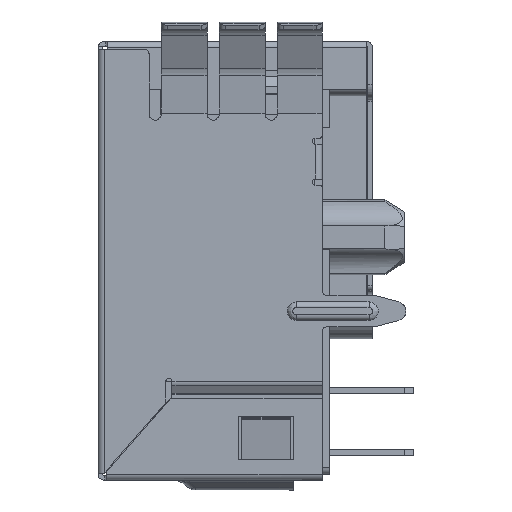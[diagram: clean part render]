
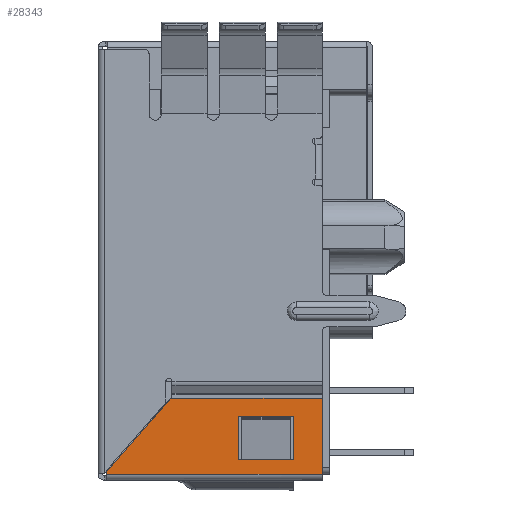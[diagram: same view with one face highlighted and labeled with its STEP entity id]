
A CAD part, left-side view. The second image highlights one B-rep face of the part: STEP entity #28343.
In plain terms, the highlighted planar face has unit normal (-1, 0, 0).
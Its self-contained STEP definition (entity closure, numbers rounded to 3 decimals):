
#635 = DIRECTION ( 'NONE',  ( 0., 0., -1. ) ) ;
#723 = DIRECTION ( 'NONE',  ( 0., 0., 1. ) ) ;
#1382 = CARTESIAN_POINT ( 'NONE',  ( -7.52, 2.664, -5.675 ) ) ;
#1685 = DIRECTION ( 'NONE',  ( 0., 1., 0. ) ) ;
#2190 = DIRECTION ( 'NONE',  ( 0., -1., 0. ) ) ;
#2287 = DIRECTION ( 'NONE',  ( 0., -0.656, 0.755 ) ) ;
#2472 = ORIENTED_EDGE ( 'NONE', *, *, #31273, .F. ) ;
#3243 = FACE_BOUND ( 'NONE', #34514, .T. ) ;
#3297 = CARTESIAN_POINT ( 'NONE',  ( -7.52, -3.595, -7.25 ) ) ;
#3355 = VERTEX_POINT ( 'NONE', #1382 ) ;
#3438 = ORIENTED_EDGE ( 'NONE', *, *, #42101, .F. ) ;
#4588 = EDGE_CURVE ( 'NONE', #16479, #9830, #34525, .T. ) ;
#4747 = ORIENTED_EDGE ( 'NONE', *, *, #38021, .F. ) ;
#5035 = VECTOR ( 'NONE', #635, 1000. ) ;
#5371 = CARTESIAN_POINT ( 'NONE',  ( -7.52, 0.86, -8.225 ) ) ;
#5658 = LINE ( 'NONE', #30235, #27336 ) ;
#8617 = LINE ( 'NONE', #3297, #37883 ) ;
#9566 = CARTESIAN_POINT ( 'NONE',  ( -7.52, 5.382, -8.802 ) ) ;
#9830 = VERTEX_POINT ( 'NONE', #13491 ) ;
#10467 = ORIENTED_EDGE ( 'NONE', *, *, #23598, .F. ) ;
#12222 = VERTEX_POINT ( 'NONE', #24461 ) ;
#12739 = VERTEX_POINT ( 'NONE', #41250 ) ;
#13322 = CARTESIAN_POINT ( 'NONE',  ( -7.52, 5.315, -8.725 ) ) ;
#13491 = CARTESIAN_POINT ( 'NONE',  ( -7.52, -3.595, -8.825 ) ) ;
#14231 = CARTESIAN_POINT ( 'NONE',  ( -7.52, -2.425, -7.25 ) ) ;
#14497 = CARTESIAN_POINT ( 'NONE',  ( -7.52, 5.315, -7.25 ) ) ;
#15833 = CARTESIAN_POINT ( 'NONE',  ( -7.52, -0.125, -6.425 ) ) ;
#16479 = VERTEX_POINT ( 'NONE', #30899 ) ;
#18339 = CARTESIAN_POINT ( 'NONE',  ( -7.52, 0.91, -8.825 ) ) ;
#19613 = VERTEX_POINT ( 'NONE', #21923 ) ;
#19682 = VERTEX_POINT ( 'NONE', #15833 ) ;
#20424 = CARTESIAN_POINT ( 'NONE',  ( -7.52, 0.86, -6.425 ) ) ;
#20758 = LINE ( 'NONE', #28058, #5035 ) ;
#21678 = LINE ( 'NONE', #9566, #28191 ) ;
#21785 = ORIENTED_EDGE ( 'NONE', *, *, #25831, .F. ) ;
#21923 = CARTESIAN_POINT ( 'NONE',  ( -7.52, -2.425, -8.225 ) ) ;
#23598 = EDGE_CURVE ( 'NONE', #12739, #19682, #28044, .T. ) ;
#24461 = CARTESIAN_POINT ( 'NONE',  ( -7.52, -3.595, -5.675 ) ) ;
#25352 = AXIS2_PLACEMENT_3D ( 'NONE', #26102, #36106, #1685 ) ;
#25679 = DIRECTION ( 'NONE',  ( 0., -1., 0. ) ) ;
#25831 = EDGE_CURVE ( 'NONE', #19613, #12739, #38801, .T. ) ;
#26102 = CARTESIAN_POINT ( 'NONE',  ( -7.52, -3.773, -8.888 ) ) ;
#26449 = VECTOR ( 'NONE', #723, 1000. ) ;
#26866 = EDGE_CURVE ( 'NONE', #19682, #30951, #20758, .T. ) ;
#27336 = VECTOR ( 'NONE', #2190, 1000. ) ;
#28044 = LINE ( 'NONE', #20424, #38394 ) ;
#28058 = CARTESIAN_POINT ( 'NONE',  ( -7.52, -0.125, -7.25 ) ) ;
#28191 = VECTOR ( 'NONE', #2287, 1000. ) ;
#28343 = ADVANCED_FACE ( 'NONE', ( #3243, #42855 ), #39617, .F. ) ;
#28553 = EDGE_CURVE ( 'NONE', #28721, #3355, #21678, .T. ) ;
#28721 = VERTEX_POINT ( 'NONE', #13322 ) ;
#29750 = EDGE_CURVE ( 'NONE', #30951, #19613, #29978, .T. ) ;
#29978 = LINE ( 'NONE', #5371, #35776 ) ;
#30235 = CARTESIAN_POINT ( 'NONE',  ( -7.52, 0.86, -5.675 ) ) ;
#30465 = DIRECTION ( 'NONE',  ( 0., 1., 0. ) ) ;
#30899 = CARTESIAN_POINT ( 'NONE',  ( -7.52, 5.315, -8.825 ) ) ;
#30951 = VERTEX_POINT ( 'NONE', #39887 ) ;
#31273 = EDGE_CURVE ( 'NONE', #12222, #9830, #8617, .T. ) ;
#31312 = LINE ( 'NONE', #14497, #26449 ) ;
#31974 = DIRECTION ( 'NONE',  ( 0., 0., 1. ) ) ;
#32594 = ORIENTED_EDGE ( 'NONE', *, *, #28553, .F. ) ;
#34514 = EDGE_LOOP ( 'NONE', ( #35483, #10467, #21785, #37379 ) ) ;
#34525 = LINE ( 'NONE', #18339, #36758 ) ;
#35483 = ORIENTED_EDGE ( 'NONE', *, *, #26866, .F. ) ;
#35776 = VECTOR ( 'NONE', #43759, 1000. ) ;
#36106 = DIRECTION ( 'NONE',  ( 1., 0., 0. ) ) ;
#36758 = VECTOR ( 'NONE', #25679, 1000. ) ;
#37095 = EDGE_LOOP ( 'NONE', ( #40130, #2472, #4747, #32594, #3438 ) ) ;
#37379 = ORIENTED_EDGE ( 'NONE', *, *, #29750, .F. ) ;
#37883 = VECTOR ( 'NONE', #44431, 1000. ) ;
#38021 = EDGE_CURVE ( 'NONE', #3355, #12222, #5658, .T. ) ;
#38394 = VECTOR ( 'NONE', #30465, 1000. ) ;
#38801 = LINE ( 'NONE', #14231, #40425 ) ;
#39617 = PLANE ( 'NONE',  #25352 ) ;
#39887 = CARTESIAN_POINT ( 'NONE',  ( -7.52, -0.125, -8.225 ) ) ;
#40130 = ORIENTED_EDGE ( 'NONE', *, *, #4588, .T. ) ;
#40425 = VECTOR ( 'NONE', #31974, 1000. ) ;
#41250 = CARTESIAN_POINT ( 'NONE',  ( -7.52, -2.425, -6.425 ) ) ;
#42101 = EDGE_CURVE ( 'NONE', #16479, #28721, #31312, .T. ) ;
#42855 = FACE_OUTER_BOUND ( 'NONE', #37095, .T. ) ;
#43759 = DIRECTION ( 'NONE',  ( 0., -1., 0. ) ) ;
#44431 = DIRECTION ( 'NONE',  ( 0., 0., -1. ) ) ;
